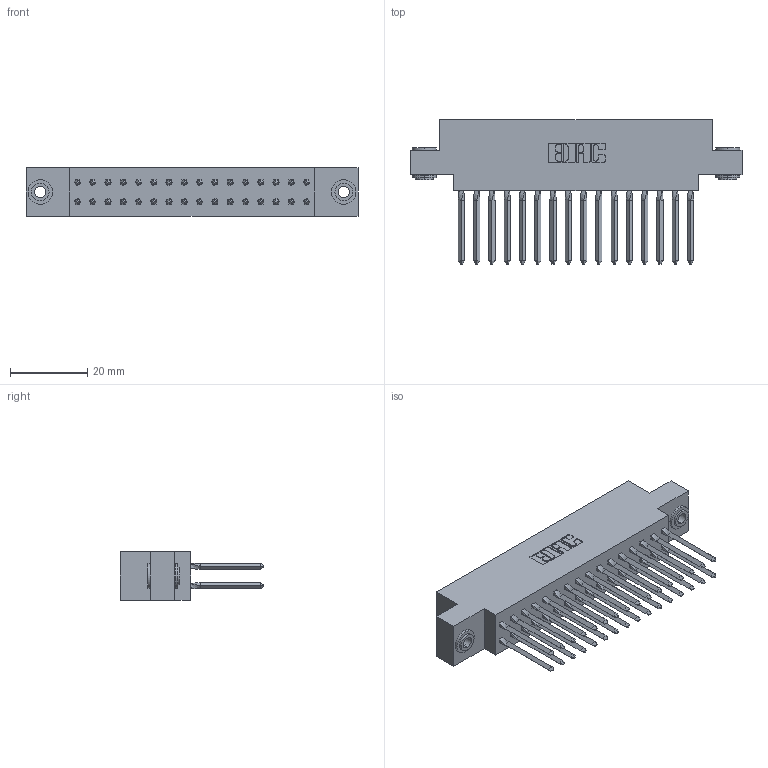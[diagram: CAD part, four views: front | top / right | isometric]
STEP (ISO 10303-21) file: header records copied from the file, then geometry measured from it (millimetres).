
FILE_DESCRIPTION (( 'STEP AP203' ), '1' );
FILE_NAME ('317-032-542-803.STEP', '2020-02-27T21:13:33', ( '' ), ( '' ), 'SwSTEP 2.0', 'SolidWorks 2016', '' );
FILE_SCHEMA (( 'CONFIG_CONTROL_DESIGN' ));
Length unit declared in the file: inch
Products named in the file (4): 317-032-542-803; 317-290-003_542; 317 Part_.156 Dia - TH; 345-250-002_345-250-002-102
Assembly tree (35 placements, depth 2):
  317-032-542-803
    317 Part_.156 Dia - TH
    317-290-003_542  x32
    345-250-002_345-250-002-102  x2
Bounding box: 86.11 x 37.34 x 12.7 mm (x, y, z)
Volume: 13297.3 mm3; surface area: 17873.1 mm2
Topology: 35 solids, 35 shells, 1964 faces, 5471 edges, 3494 vertices
Faces by surface type: plane 1540, cylinder 288, bspline 128, cone 8
Entity records: 26422 total; most frequent: CARTESIAN_POINT 4824, ORIENTED_EDGE 4480, DIRECTION 3854, EDGE_CURVE 2240, LINE 2046, VECTOR 2046, VERTEX_POINT 1486, AXIS2_PLACEMENT_3D 904
